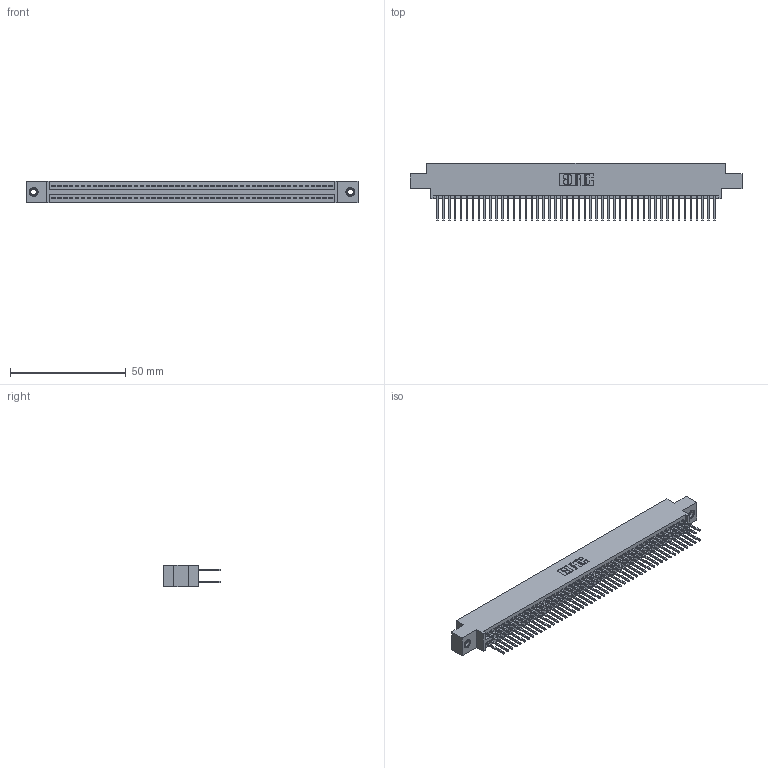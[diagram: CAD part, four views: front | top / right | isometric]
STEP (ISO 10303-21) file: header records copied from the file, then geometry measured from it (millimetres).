
FILE_DESCRIPTION (( 'STEP AP203' ), '1' );
FILE_NAME ('345-096-523-807.STEP', '2019-11-02T07:20:44', ( '' ), ( '' ), 'SwSTEP 2.0', 'SolidWorks 2016', '' );
FILE_SCHEMA (( 'CONFIG_CONTROL_DESIGN' ));
Length unit declared in the file: inch
Products named in the file (4): 345 Part_0.170 Offset - 0.156 Dia-TI; 345-250-001_345-250-005-103; 345-292-001_345-293-123; 345-096-523-807
Assembly tree (99 placements, depth 2):
  345-096-523-807
    345 Part_0.170 Offset - 0.156 Dia-TI
    345-292-001_345-293-123  x96
    345-250-001_345-250-005-103  x2
Bounding box: 143.13 x 24.82 x 9.4 mm (x, y, z)
Volume: 14029.3 mm3; surface area: 21907.8 mm2
Topology: 99 solids, 99 shells, 4990 faces, 14793 edges, 9726 vertices
Faces by surface type: plane 3284, cylinder 1690, cone 12, torus 4
Entity records: 38190 total; most frequent: CARTESIAN_POINT 6379, ORIENTED_EDGE 6306, DIRECTION 5643, EDGE_CURVE 3153, VECTOR 2809, LINE 2809, VERTEX_POINT 2096, AXIS2_PLACEMENT_3D 1417
